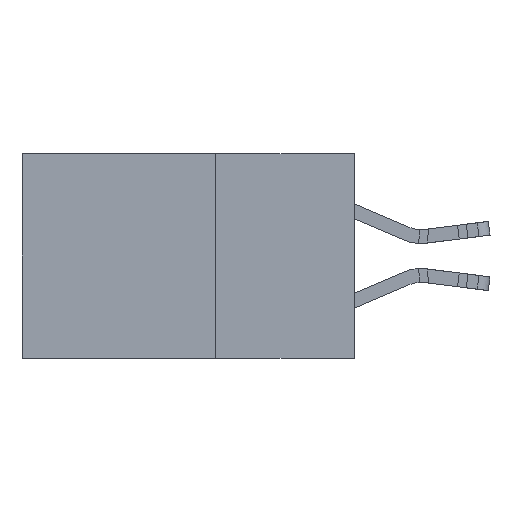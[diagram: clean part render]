
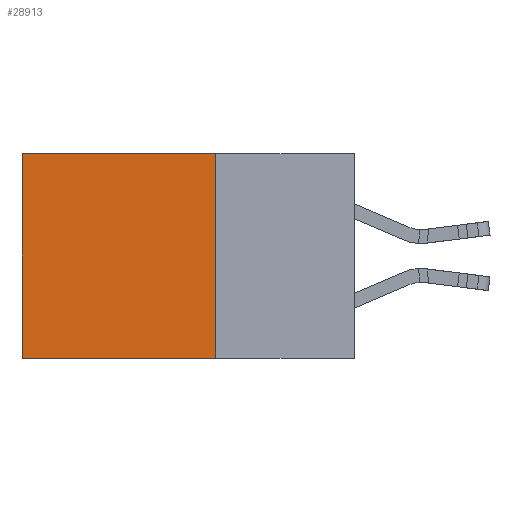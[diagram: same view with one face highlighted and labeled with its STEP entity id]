
A CAD part, left-side view. The second image highlights one B-rep face of the part: STEP entity #28913.
In plain terms, the highlighted planar face has unit normal (-1, 0, 0).
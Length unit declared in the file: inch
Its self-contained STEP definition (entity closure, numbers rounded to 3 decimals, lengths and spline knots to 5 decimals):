
#52 = CARTESIAN_POINT ( 'NONE',  ( 0.298, 0.6, 0. ) ) ;
#273 = AXIS2_PLACEMENT_3D ( 'NONE', #25043, #11584, #27313 ) ;
#656 = DIRECTION ( 'NONE',  ( 0., 0., -1. ) ) ;
#1221 = CARTESIAN_POINT ( 'NONE',  ( 0.298, 0.6, 0. ) ) ;
#1387 = EDGE_LOOP ( 'NONE', ( #20592, #21099, #22384, #27792 ) ) ;
#2797 = EDGE_CURVE ( 'NONE', #21789, #23313, #6273, .T. ) ;
#4231 = LINE ( 'NONE', #14638, #15802 ) ;
#5529 = EDGE_CURVE ( 'NONE', #26589, #28338, #25746, .T. ) ;
#5868 = CARTESIAN_POINT ( 'NONE',  ( 0.298, 0.25, -0.37 ) ) ;
#6273 = LINE ( 'NONE', #29203, #12430 ) ;
#6931 = PLANE ( 'NONE',  #273 ) ;
#8532 = VECTOR ( 'NONE', #19665, 39.37008 ) ;
#11584 = DIRECTION ( 'NONE',  ( 1., 0., 0. ) ) ;
#12224 = EDGE_CURVE ( 'NONE', #23313, #28338, #15341, .T. ) ;
#12430 = VECTOR ( 'NONE', #29517, 39.37008 ) ;
#14638 = CARTESIAN_POINT ( 'NONE',  ( 0.298, 0.25, 0. ) ) ;
#15341 = LINE ( 'NONE', #1221, #8532 ) ;
#15802 = VECTOR ( 'NONE', #656, 39.37008 ) ;
#15829 = FACE_OUTER_BOUND ( 'NONE', #1387, .T. ) ;
#17375 = CARTESIAN_POINT ( 'NONE',  ( 0.298, 0.25, 0. ) ) ;
#19665 = DIRECTION ( 'NONE',  ( 0., 0., -1. ) ) ;
#19796 = VECTOR ( 'NONE', #21881, 39.37008 ) ;
#20592 = ORIENTED_EDGE ( 'NONE', *, *, #12224, .T. ) ;
#21099 = ORIENTED_EDGE ( 'NONE', *, *, #5529, .F. ) ;
#21789 = VERTEX_POINT ( 'NONE', #17375 ) ;
#21881 = DIRECTION ( 'NONE',  ( 0., 1., 0. ) ) ;
#22384 = ORIENTED_EDGE ( 'NONE', *, *, #23511, .F. ) ;
#23011 = CARTESIAN_POINT ( 'NONE',  ( 0.298, 0.6, -0.37 ) ) ;
#23313 = VERTEX_POINT ( 'NONE', #52 ) ;
#23351 = CARTESIAN_POINT ( 'NONE',  ( 0.298, 0.25, -0.37 ) ) ;
#23511 = EDGE_CURVE ( 'NONE', #21789, #26589, #4231, .T. ) ;
#25043 = CARTESIAN_POINT ( 'NONE',  ( 0.298, 0.25, 0. ) ) ;
#25746 = LINE ( 'NONE', #5868, #19796 ) ;
#26589 = VERTEX_POINT ( 'NONE', #23351 ) ;
#27313 = DIRECTION ( 'NONE',  ( 0., 0., -1. ) ) ;
#27792 = ORIENTED_EDGE ( 'NONE', *, *, #2797, .T. ) ;
#28338 = VERTEX_POINT ( 'NONE', #23011 ) ;
#28913 = ADVANCED_FACE ( 'NONE', ( #15829 ), #6931, .F. ) ;
#29203 = CARTESIAN_POINT ( 'NONE',  ( 0.298, 0.25, 0. ) ) ;
#29517 = DIRECTION ( 'NONE',  ( 0., 1., 0. ) ) ;
